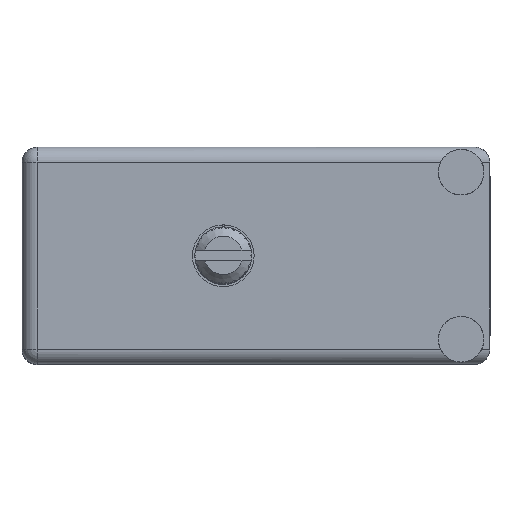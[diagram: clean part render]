
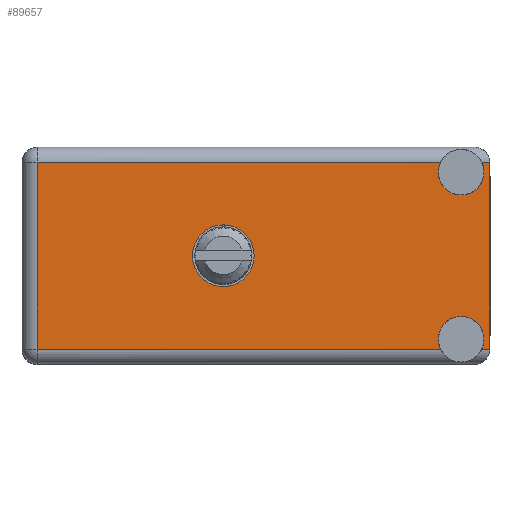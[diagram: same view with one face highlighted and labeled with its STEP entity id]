
A CAD part, top view. The second image highlights one B-rep face of the part: STEP entity #89657.
In plain terms, the highlighted face is planar.
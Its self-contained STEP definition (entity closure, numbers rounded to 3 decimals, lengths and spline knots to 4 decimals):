
#5355 = EDGE_CURVE ( 'NONE', #83274, #34816, #23183, .T. ) ;
#5928 = DIRECTION ( 'NONE',  ( 0., 1., 0. ) ) ;
#6975 = DIRECTION ( 'NONE',  ( 1., 0., 0. ) ) ;
#9998 = CIRCLE ( 'NONE', #151720, 0.075 ) ;
#10214 = CARTESIAN_POINT ( 'NONE',  ( 1.539, 0.906, 0. ) ) ;
#11462 = VERTEX_POINT ( 'NONE', #91493 ) ;
#12618 = DIRECTION ( 'NONE',  ( 0., 0., 1. ) ) ;
#14091 = ORIENTED_EDGE ( 'NONE', *, *, #147825, .T. ) ;
#15866 = VECTOR ( 'NONE', #6975, 39.3701 ) ;
#16356 = DIRECTION ( 'NONE',  ( 0., 1., 0. ) ) ;
#19160 = EDGE_LOOP ( 'NONE', ( #59401, #98786 ) ) ;
#20132 = ORIENTED_EDGE ( 'NONE', *, *, #74869, .T. ) ;
#21950 = EDGE_CURVE ( 'NONE', #164752, #11462, #9998, .T. ) ;
#23183 = CIRCLE ( 'NONE', #85017, 0.1015 ) ;
#23671 = DIRECTION ( 'NONE',  ( 0., 1., 0. ) ) ;
#24676 = VERTEX_POINT ( 'NONE', #125972 ) ;
#26975 = LINE ( 'NONE', #52736, #55587 ) ;
#30019 = EDGE_LOOP ( 'NONE', ( #54420, #119483, #133801, #120359, #46741, #20132, #38818, #119075, #14091, #111157 ) ) ;
#32293 = CARTESIAN_POINT ( 'NONE',  ( 0.05, 0.906, -0.665 ) ) ;
#33887 = EDGE_CURVE ( 'NONE', #66468, #63431, #65774, .T. ) ;
#34816 = VERTEX_POINT ( 'NONE', #159984 ) ;
#37011 = CARTESIAN_POINT ( 'NONE',  ( 0.05, 0.906, -0.715 ) ) ;
#37559 = LINE ( 'NONE', #101980, #77012 ) ;
#38818 = ORIENTED_EDGE ( 'NONE', *, *, #106312, .F. ) ;
#39378 = VERTEX_POINT ( 'NONE', #71608 ) ;
#40203 = CARTESIAN_POINT ( 'NONE',  ( 1.445, 0.906, -0.6325 ) ) ;
#46067 = CARTESIAN_POINT ( 'NONE',  ( 1.445, 0.906, -0.0825 ) ) ;
#46741 = ORIENTED_EDGE ( 'NONE', *, *, #71759, .F. ) ;
#48177 = DIRECTION ( 'NONE',  ( 0., 0., 1. ) ) ;
#48394 = VERTEX_POINT ( 'NONE', #153217 ) ;
#49193 = CARTESIAN_POINT ( 'NONE',  ( 1.445, 0.906, -0.6325 ) ) ;
#52736 = CARTESIAN_POINT ( 'NONE',  ( 1.539, 0.906, -0.05 ) ) ;
#54420 = ORIENTED_EDGE ( 'NONE', *, *, #176017, .T. ) ;
#55587 = VECTOR ( 'NONE', #110859, 39.3701 ) ;
#55967 = DIRECTION ( 'NONE',  ( 0., 0., 1. ) ) ;
#56189 = DIRECTION ( 'NONE',  ( 0., 0., 1. ) ) ;
#58330 = VERTEX_POINT ( 'NONE', #142921 ) ;
#59401 = ORIENTED_EDGE ( 'NONE', *, *, #74808, .F. ) ;
#63431 = VERTEX_POINT ( 'NONE', #67635 ) ;
#65774 = CIRCLE ( 'NONE', #115889, 0.075 ) ;
#66468 = VERTEX_POINT ( 'NONE', #138835 ) ;
#67635 = CARTESIAN_POINT ( 'NONE',  ( 1.445, 0.906, -0.5575 ) ) ;
#69781 = VECTOR ( 'NONE', #130422, 39.3701 ) ;
#70709 = CARTESIAN_POINT ( 'NONE',  ( 1.5126, 0.906, -0.05 ) ) ;
#70806 = VECTOR ( 'NONE', #56189, 39.3701 ) ;
#70945 = DIRECTION ( 'NONE',  ( 0., 0., 1. ) ) ;
#71608 = CARTESIAN_POINT ( 'NONE',  ( 1.539, 0.906, -0.665 ) ) ;
#71759 = EDGE_CURVE ( 'NONE', #39378, #58330, #109749, .T. ) ;
#73518 = AXIS2_PLACEMENT_3D ( 'NONE', #46067, #142899, #70945 ) ;
#74808 = EDGE_CURVE ( 'NONE', #34816, #83274, #147714, .T. ) ;
#74869 = EDGE_CURVE ( 'NONE', #39378, #48394, #37559, .T. ) ;
#75813 = CARTESIAN_POINT ( 'NONE',  ( 1.445, 0.906, -0.0825 ) ) ;
#76550 = CIRCLE ( 'NONE', #73518, 0.075 ) ;
#76736 = DIRECTION ( 'NONE',  ( 0., 1., 0. ) ) ;
#77012 = VECTOR ( 'NONE', #87229, 39.3701 ) ;
#83274 = VERTEX_POINT ( 'NONE', #84629 ) ;
#84629 = CARTESIAN_POINT ( 'NONE',  ( 0.6625, 0.906, -0.459 ) ) ;
#85017 = AXIS2_PLACEMENT_3D ( 'NONE', #156504, #16356, #55967 ) ;
#85061 = CARTESIAN_POINT ( 'NONE',  ( 1.3774, 0.906, -0.05 ) ) ;
#87229 = DIRECTION ( 'NONE',  ( -1., 0., 0. ) ) ;
#89657 = ADVANCED_FACE ( 'NONE', ( #151120, #152956 ), #167715, .T. ) ;
#91493 = CARTESIAN_POINT ( 'NONE',  ( 1.445, 0.906, -0.1575 ) ) ;
#92033 = EDGE_CURVE ( 'NONE', #162867, #24676, #95041, .T. ) ;
#95041 = LINE ( 'NONE', #37011, #180056 ) ;
#96447 = DIRECTION ( 'NONE',  ( 0., 0., 1. ) ) ;
#98786 = ORIENTED_EDGE ( 'NONE', *, *, #5355, .F. ) ;
#101980 = CARTESIAN_POINT ( 'NONE',  ( 0., 0.906, -0.665 ) ) ;
#106312 = EDGE_CURVE ( 'NONE', #63431, #48394, #163152, .T. ) ;
#109290 = AXIS2_PLACEMENT_3D ( 'NONE', #109651, #126205, #137307 ) ;
#109651 = CARTESIAN_POINT ( 'NONE',  ( 0., 0.906, -0.715 ) ) ;
#109749 = LINE ( 'NONE', #10214, #70806 ) ;
#110859 = DIRECTION ( 'NONE',  ( 1., 0., 0. ) ) ;
#111157 = ORIENTED_EDGE ( 'NONE', *, *, #92033, .T. ) ;
#111271 = VERTEX_POINT ( 'NONE', #85061 ) ;
#115889 = AXIS2_PLACEMENT_3D ( 'NONE', #40203, #23671, #96447 ) ;
#119075 = ORIENTED_EDGE ( 'NONE', *, *, #33887, .F. ) ;
#119483 = ORIENTED_EDGE ( 'NONE', *, *, #173575, .F. ) ;
#119847 = EDGE_CURVE ( 'NONE', #164752, #58330, #133259, .T. ) ;
#120359 = ORIENTED_EDGE ( 'NONE', *, *, #119847, .T. ) ;
#121283 = AXIS2_PLACEMENT_3D ( 'NONE', #124192, #152749, #12618 ) ;
#124192 = CARTESIAN_POINT ( 'NONE',  ( 0.6625, 0.906, -0.3575 ) ) ;
#125972 = CARTESIAN_POINT ( 'NONE',  ( 0.05, 0.906, -0.05 ) ) ;
#126205 = DIRECTION ( 'NONE',  ( 0., 1., 0. ) ) ;
#127709 = LINE ( 'NONE', #128619, #69781 ) ;
#128619 = CARTESIAN_POINT ( 'NONE',  ( 0., 0.906, -0.665 ) ) ;
#130422 = DIRECTION ( 'NONE',  ( -1., 0., 0. ) ) ;
#133259 = LINE ( 'NONE', #176520, #15866 ) ;
#133801 = ORIENTED_EDGE ( 'NONE', *, *, #21950, .F. ) ;
#134727 = DIRECTION ( 'NONE',  ( 0., 0., 1. ) ) ;
#137307 = DIRECTION ( 'NONE',  ( 0., 0., 1. ) ) ;
#138835 = CARTESIAN_POINT ( 'NONE',  ( 1.3774, 0.906, -0.665 ) ) ;
#142523 = AXIS2_PLACEMENT_3D ( 'NONE', #49193, #5928, #175498 ) ;
#142899 = DIRECTION ( 'NONE',  ( 0., 1., 0. ) ) ;
#142921 = CARTESIAN_POINT ( 'NONE',  ( 1.539, 0.906, -0.05 ) ) ;
#147714 = CIRCLE ( 'NONE', #121283, 0.1015 ) ;
#147825 = EDGE_CURVE ( 'NONE', #66468, #162867, #127709, .T. ) ;
#151120 = FACE_BOUND ( 'NONE', #19160, .T. ) ;
#151720 = AXIS2_PLACEMENT_3D ( 'NONE', #75813, #76736, #48177 ) ;
#152749 = DIRECTION ( 'NONE',  ( 0., 1., 0. ) ) ;
#152956 = FACE_OUTER_BOUND ( 'NONE', #30019, .T. ) ;
#153217 = CARTESIAN_POINT ( 'NONE',  ( 1.5126, 0.906, -0.665 ) ) ;
#156504 = CARTESIAN_POINT ( 'NONE',  ( 0.6625, 0.906, -0.3575 ) ) ;
#159984 = CARTESIAN_POINT ( 'NONE',  ( 0.6625, 0.906, -0.256 ) ) ;
#162867 = VERTEX_POINT ( 'NONE', #32293 ) ;
#163152 = CIRCLE ( 'NONE', #142523, 0.075 ) ;
#164752 = VERTEX_POINT ( 'NONE', #70709 ) ;
#167715 = PLANE ( 'NONE',  #109290 ) ;
#173575 = EDGE_CURVE ( 'NONE', #11462, #111271, #76550, .T. ) ;
#175498 = DIRECTION ( 'NONE',  ( 0., 0., 1. ) ) ;
#176017 = EDGE_CURVE ( 'NONE', #24676, #111271, #26975, .T. ) ;
#176520 = CARTESIAN_POINT ( 'NONE',  ( 1.539, 0.906, -0.05 ) ) ;
#180056 = VECTOR ( 'NONE', #134727, 39.3701 ) ;
